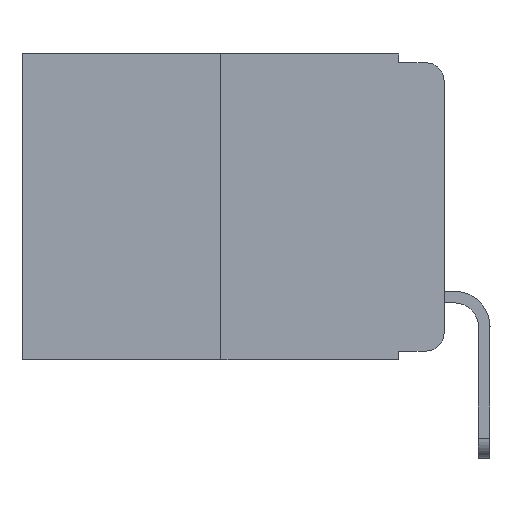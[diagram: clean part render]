
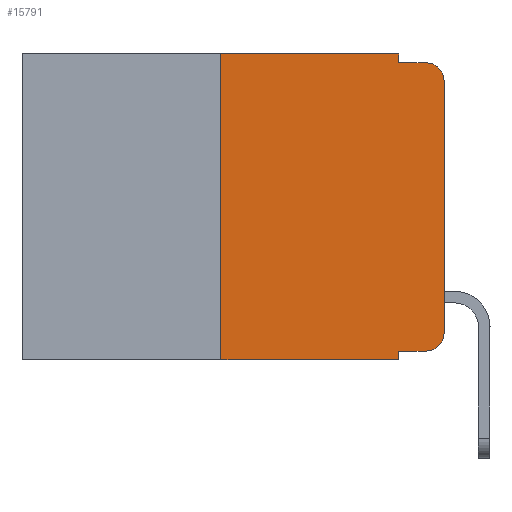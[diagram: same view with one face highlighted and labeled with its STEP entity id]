
A CAD part, left-side view. The second image highlights one B-rep face of the part: STEP entity #15791.
In plain terms, the highlighted planar face has unit normal (-1, 0, 0).
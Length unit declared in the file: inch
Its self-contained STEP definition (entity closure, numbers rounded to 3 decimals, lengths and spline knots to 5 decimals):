
#329 = DIRECTION ( 'NONE',  ( 0., 0., 1. ) ) ;
#337 = VECTOR ( 'NONE', #9453, 39.37008 ) ;
#688 = DIRECTION ( 'NONE',  ( -1., 0., 0. ) ) ;
#709 = AXIS2_PLACEMENT_3D ( 'NONE', #15631, #688, #11018 ) ;
#727 = AXIS2_PLACEMENT_3D ( 'NONE', #16695, #13592, #8902 ) ;
#767 = CARTESIAN_POINT ( 'NONE',  ( 0., 0.051, 0. ) ) ;
#856 = CARTESIAN_POINT ( 'NONE',  ( 0., 0.051, -0.333 ) ) ;
#877 = DIRECTION ( 'NONE',  ( 0., -1., 0. ) ) ;
#975 = DIRECTION ( 'NONE',  ( -1., 0., 0. ) ) ;
#1506 = DIRECTION ( 'NONE',  ( 0., 0., -1. ) ) ;
#1782 = EDGE_CURVE ( 'NONE', #9691, #9324, #4605, .T. ) ;
#1999 = DIRECTION ( 'NONE',  ( 0., 0., -1. ) ) ;
#2074 = CARTESIAN_POINT ( 'NONE',  ( 0., 0.051, -0.343 ) ) ;
#2512 = VERTEX_POINT ( 'NONE', #2074 ) ;
#2677 = CARTESIAN_POINT ( 'NONE',  ( 0., 0.473, -0.343 ) ) ;
#2834 = EDGE_CURVE ( 'NONE', #8125, #7100, #8985, .T. ) ;
#2857 = ORIENTED_EDGE ( 'NONE', *, *, #2834, .F. ) ;
#3135 = ORIENTED_EDGE ( 'NONE', *, *, #8999, .T. ) ;
#3267 = DIRECTION ( 'NONE',  ( 0., 0., 1. ) ) ;
#3302 = VECTOR ( 'NONE', #1506, 39.37008 ) ;
#4605 = LINE ( 'NONE', #12022, #10988 ) ;
#4963 = VERTEX_POINT ( 'NONE', #9240 ) ;
#5132 = ORIENTED_EDGE ( 'NONE', *, *, #15670, .T. ) ;
#5199 = CARTESIAN_POINT ( 'NONE',  ( 0., 0.473, 0. ) ) ;
#5630 = VECTOR ( 'NONE', #1999, 39.37008 ) ;
#5781 = VECTOR ( 'NONE', #8712, 39.37008 ) ;
#6194 = ORIENTED_EDGE ( 'NONE', *, *, #11330, .F. ) ;
#6449 = CARTESIAN_POINT ( 'NONE',  ( 0., 0.02, -0.333 ) ) ;
#6855 = CARTESIAN_POINT ( 'NONE',  ( 0., 0., -0.03 ) ) ;
#7100 = VERTEX_POINT ( 'NONE', #14385 ) ;
#8125 = VERTEX_POINT ( 'NONE', #11626 ) ;
#8149 = LINE ( 'NONE', #5199, #337 ) ;
#8416 = LINE ( 'NONE', #14494, #10886 ) ;
#8502 = DIRECTION ( 'NONE',  ( 0., 0., -1. ) ) ;
#8529 = ORIENTED_EDGE ( 'NONE', *, *, #17136, .F. ) ;
#8712 = DIRECTION ( 'NONE',  ( 0., -1., 0. ) ) ;
#8902 = DIRECTION ( 'NONE',  ( 0., 0., -1. ) ) ;
#8914 = ORIENTED_EDGE ( 'NONE', *, *, #15479, .T. ) ;
#8985 = LINE ( 'NONE', #10676, #9499 ) ;
#8999 = EDGE_CURVE ( 'NONE', #9324, #4963, #11369, .T. ) ;
#9240 = CARTESIAN_POINT ( 'NONE',  ( 0., 0.02, -0.01 ) ) ;
#9275 = ORIENTED_EDGE ( 'NONE', *, *, #11558, .F. ) ;
#9324 = VERTEX_POINT ( 'NONE', #6855 ) ;
#9453 = DIRECTION ( 'NONE',  ( 0., -1., 0. ) ) ;
#9499 = VECTOR ( 'NONE', #3267, 39.37008 ) ;
#9691 = VERTEX_POINT ( 'NONE', #13203 ) ;
#10014 = VERTEX_POINT ( 'NONE', #6449 ) ;
#10236 = LINE ( 'NONE', #17919, #14928 ) ;
#10532 = DIRECTION ( 'NONE',  ( 0., -1., 0. ) ) ;
#10676 = CARTESIAN_POINT ( 'NONE',  ( 0., 0.25, 0. ) ) ;
#10886 = VECTOR ( 'NONE', #877, 39.37008 ) ;
#10926 = CARTESIAN_POINT ( 'NONE',  ( 0., 0.051, -0.01 ) ) ;
#10988 = VECTOR ( 'NONE', #329, 39.37008 ) ;
#11018 = DIRECTION ( 'NONE',  ( 0., 0., -1. ) ) ;
#11330 = EDGE_CURVE ( 'NONE', #7100, #15144, #8149, .T. ) ;
#11369 = CIRCLE ( 'NONE', #13941, 0.02 ) ;
#11400 = ORIENTED_EDGE ( 'NONE', *, *, #14088, .F. ) ;
#11558 = EDGE_CURVE ( 'NONE', #13027, #4963, #10236, .T. ) ;
#11626 = CARTESIAN_POINT ( 'NONE',  ( 0., 0.25, -0.343 ) ) ;
#11699 = ORIENTED_EDGE ( 'NONE', *, *, #15614, .T. ) ;
#12022 = CARTESIAN_POINT ( 'NONE',  ( 0., 0., 0. ) ) ;
#13027 = VERTEX_POINT ( 'NONE', #10926 ) ;
#13100 = LINE ( 'NONE', #2677, #5781 ) ;
#13203 = CARTESIAN_POINT ( 'NONE',  ( 0., 0., -0.313 ) ) ;
#13529 = VERTEX_POINT ( 'NONE', #856 ) ;
#13592 = DIRECTION ( 'NONE',  ( 1., 0., 0. ) ) ;
#13701 = FACE_OUTER_BOUND ( 'NONE', #15781, .T. ) ;
#13941 = AXIS2_PLACEMENT_3D ( 'NONE', #16083, #975, #8502 ) ;
#14088 = EDGE_CURVE ( 'NONE', #13529, #2512, #18108, .T. ) ;
#14385 = CARTESIAN_POINT ( 'NONE',  ( 0., 0.25, 0. ) ) ;
#14494 = CARTESIAN_POINT ( 'NONE',  ( 0., 0.051, -0.333 ) ) ;
#14813 = CARTESIAN_POINT ( 'NONE',  ( 0., 0.051, 0. ) ) ;
#14928 = VECTOR ( 'NONE', #10532, 39.37008 ) ;
#15144 = VERTEX_POINT ( 'NONE', #14813 ) ;
#15349 = CIRCLE ( 'NONE', #709, 0.02 ) ;
#15479 = EDGE_CURVE ( 'NONE', #10014, #9691, #15349, .T. ) ;
#15614 = EDGE_CURVE ( 'NONE', #8125, #2512, #13100, .T. ) ;
#15631 = CARTESIAN_POINT ( 'NONE',  ( 0., 0.02, -0.313 ) ) ;
#15670 = EDGE_CURVE ( 'NONE', #13529, #10014, #8416, .T. ) ;
#15781 = EDGE_LOOP ( 'NONE', ( #16240, #3135, #9275, #8529, #6194, #2857, #11699, #11400, #5132, #8914 ) ) ;
#15791 = ADVANCED_FACE ( 'NONE', ( #13701 ), #18090, .F. ) ;
#16083 = CARTESIAN_POINT ( 'NONE',  ( 0., 0.02, -0.03 ) ) ;
#16240 = ORIENTED_EDGE ( 'NONE', *, *, #1782, .T. ) ;
#16515 = CARTESIAN_POINT ( 'NONE',  ( 0., 0.051, 0. ) ) ;
#16695 = CARTESIAN_POINT ( 'NONE',  ( 0., 0.473, 0. ) ) ;
#17136 = EDGE_CURVE ( 'NONE', #15144, #13027, #17385, .T. ) ;
#17385 = LINE ( 'NONE', #767, #5630 ) ;
#17919 = CARTESIAN_POINT ( 'NONE',  ( 0., 0.051, -0.01 ) ) ;
#18090 = PLANE ( 'NONE',  #727 ) ;
#18108 = LINE ( 'NONE', #16515, #3302 ) ;
